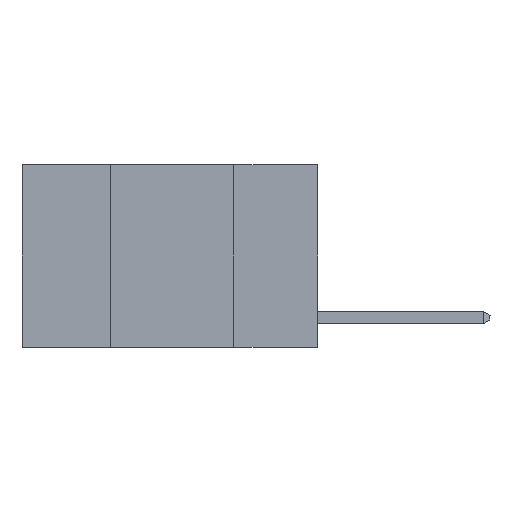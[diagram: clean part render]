
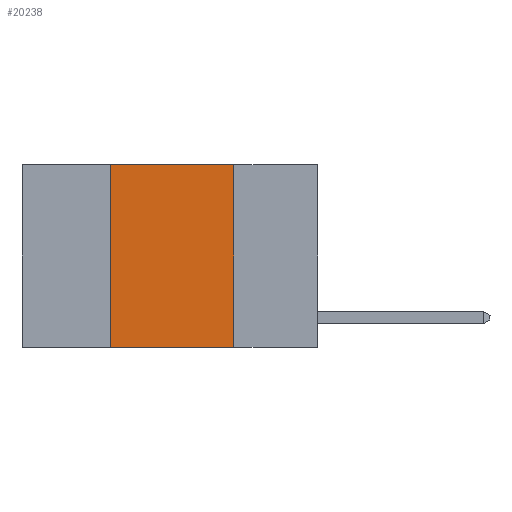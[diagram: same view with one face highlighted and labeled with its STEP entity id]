
A CAD part, left-side view. The second image highlights one B-rep face of the part: STEP entity #20238.
In plain terms, the highlighted planar face has unit normal (-1, 0, 0).
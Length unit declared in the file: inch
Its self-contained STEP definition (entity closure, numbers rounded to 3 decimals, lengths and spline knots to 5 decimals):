
#380 = AXIS2_PLACEMENT_3D ( 'NONE', #5084, #13347, #9168 ) ;
#774 = VECTOR ( 'NONE', #24433, 39.37008 ) ;
#832 = ORIENTED_EDGE ( 'NONE', *, *, #17234, .F. ) ;
#3162 = VERTEX_POINT ( 'NONE', #21521 ) ;
#4461 = LINE ( 'NONE', #10388, #12485 ) ;
#4609 = DIRECTION ( 'NONE',  ( 0., -1., 0. ) ) ;
#5084 = CARTESIAN_POINT ( 'NONE',  ( 0., 0.6, 0. ) ) ;
#5202 = CARTESIAN_POINT ( 'NONE',  ( 0., 0.6, -0.37 ) ) ;
#6894 = LINE ( 'NONE', #5202, #7580 ) ;
#6920 = VERTEX_POINT ( 'NONE', #18724 ) ;
#7580 = VECTOR ( 'NONE', #23808, 39.37008 ) ;
#8646 = CARTESIAN_POINT ( 'NONE',  ( 0., 0.6, 0. ) ) ;
#9168 = DIRECTION ( 'NONE',  ( 0., 0., -1. ) ) ;
#10388 = CARTESIAN_POINT ( 'NONE',  ( 0., 0.17, 0. ) ) ;
#12485 = VECTOR ( 'NONE', #26620, 39.37008 ) ;
#12970 = VERTEX_POINT ( 'NONE', #23333 ) ;
#13347 = DIRECTION ( 'NONE',  ( 1., 0., 0. ) ) ;
#13764 = ORIENTED_EDGE ( 'NONE', *, *, #16978, .T. ) ;
#14046 = EDGE_CURVE ( 'NONE', #3162, #12970, #26445, .T. ) ;
#14320 = ORIENTED_EDGE ( 'NONE', *, *, #15155, .F. ) ;
#15155 = EDGE_CURVE ( 'NONE', #12970, #6920, #4461, .T. ) ;
#15246 = PLANE ( 'NONE',  #380 ) ;
#16261 = LINE ( 'NONE', #22535, #774 ) ;
#16978 = EDGE_CURVE ( 'NONE', #22342, #6920, #6894, .T. ) ;
#17234 = EDGE_CURVE ( 'NONE', #22342, #3162, #16261, .T. ) ;
#18724 = CARTESIAN_POINT ( 'NONE',  ( 0., 0.17, -0.37 ) ) ;
#19236 = CARTESIAN_POINT ( 'NONE',  ( 0., 0.42, -0.37 ) ) ;
#20238 = ADVANCED_FACE ( 'NONE', ( #25388 ), #15246, .F. ) ;
#20678 = ORIENTED_EDGE ( 'NONE', *, *, #14046, .F. ) ;
#21283 = EDGE_LOOP ( 'NONE', ( #14320, #20678, #832, #13764 ) ) ;
#21521 = CARTESIAN_POINT ( 'NONE',  ( 0., 0.42, 0. ) ) ;
#22342 = VERTEX_POINT ( 'NONE', #19236 ) ;
#22535 = CARTESIAN_POINT ( 'NONE',  ( 0., 0.42, 0. ) ) ;
#23333 = CARTESIAN_POINT ( 'NONE',  ( 0., 0.17, 0. ) ) ;
#23808 = DIRECTION ( 'NONE',  ( 0., -1., 0. ) ) ;
#24433 = DIRECTION ( 'NONE',  ( 0., 0., 1. ) ) ;
#25388 = FACE_OUTER_BOUND ( 'NONE', #21283, .T. ) ;
#25455 = VECTOR ( 'NONE', #4609, 39.37008 ) ;
#26445 = LINE ( 'NONE', #8646, #25455 ) ;
#26620 = DIRECTION ( 'NONE',  ( 0., 0., -1. ) ) ;
